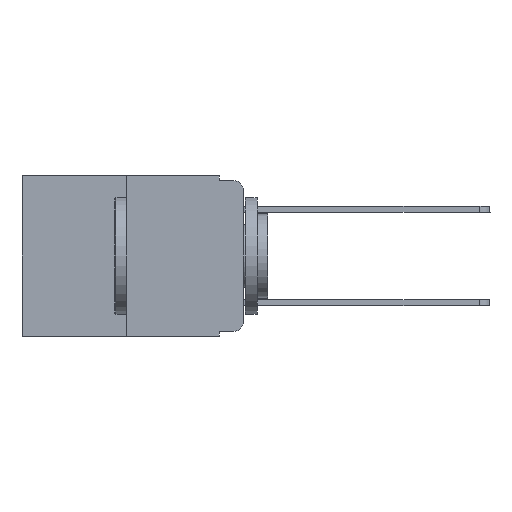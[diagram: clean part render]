
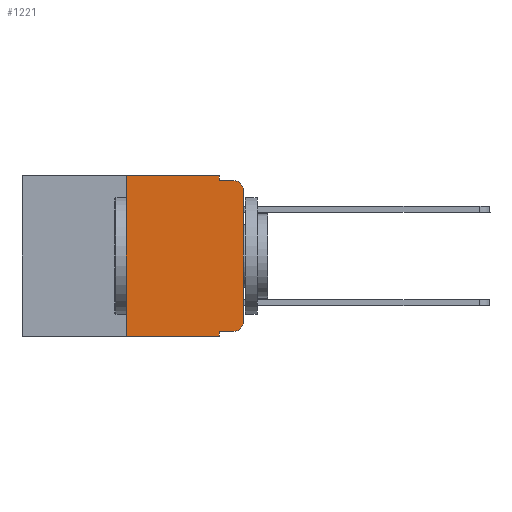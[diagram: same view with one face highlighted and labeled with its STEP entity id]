
A CAD part, left-side view. The second image highlights one B-rep face of the part: STEP entity #1221.
In plain terms, the highlighted planar face has unit normal (-1, 0, 0).
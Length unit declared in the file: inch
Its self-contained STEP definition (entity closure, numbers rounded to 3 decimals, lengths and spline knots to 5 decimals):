
#422 = AXIS2_PLACEMENT_3D ( 'NONE', #8731, #4426, #17679 ) ;
#542 = CARTESIAN_POINT ( 'NONE',  ( 0., 0.02, -0.333 ) ) ;
#1221 = ADVANCED_FACE ( 'NONE', ( #9738 ), #8747, .F. ) ;
#1279 = VERTEX_POINT ( 'NONE', #10726 ) ;
#1606 = CARTESIAN_POINT ( 'NONE',  ( 0., 0.473, -0.343 ) ) ;
#2159 = VERTEX_POINT ( 'NONE', #2429 ) ;
#2238 = ORIENTED_EDGE ( 'NONE', *, *, #3857, .T. ) ;
#2368 = DIRECTION ( 'NONE',  ( -1., 0., 0. ) ) ;
#2429 = CARTESIAN_POINT ( 'NONE',  ( 0., 0.051, -0.343 ) ) ;
#2742 = VERTEX_POINT ( 'NONE', #5523 ) ;
#2778 = LINE ( 'NONE', #15766, #17876 ) ;
#3284 = ORIENTED_EDGE ( 'NONE', *, *, #5958, .T. ) ;
#3495 = EDGE_CURVE ( 'NONE', #1279, #2742, #3902, .T. ) ;
#3747 = EDGE_CURVE ( 'NONE', #4686, #7341, #6860, .T. ) ;
#3857 = EDGE_CURVE ( 'NONE', #1279, #2159, #15197, .T. ) ;
#3902 = LINE ( 'NONE', #12713, #14790 ) ;
#4000 = ORIENTED_EDGE ( 'NONE', *, *, #8654, .F. ) ;
#4116 = VECTOR ( 'NONE', #4656, 39.37008 ) ;
#4294 = VECTOR ( 'NONE', #17960, 39.37008 ) ;
#4426 = DIRECTION ( 'NONE',  ( -1., 0., 0. ) ) ;
#4656 = DIRECTION ( 'NONE',  ( 0., 0., 1. ) ) ;
#4686 = VERTEX_POINT ( 'NONE', #17404 ) ;
#4939 = ORIENTED_EDGE ( 'NONE', *, *, #3747, .F. ) ;
#4977 = EDGE_LOOP ( 'NONE', ( #18023, #12356, #4939, #4000, #7674, #10097, #2238, #9635, #3284, #13152 ) ) ;
#5523 = CARTESIAN_POINT ( 'NONE',  ( 0., 0.25, 0. ) ) ;
#5594 = VECTOR ( 'NONE', #13557, 39.37008 ) ;
#5663 = DIRECTION ( 'NONE',  ( 0., -1., 0. ) ) ;
#5920 = VECTOR ( 'NONE', #16324, 39.37008 ) ;
#5958 = EDGE_CURVE ( 'NONE', #7833, #14600, #10935, .T. ) ;
#6187 = EDGE_CURVE ( 'NONE', #2742, #14765, #11849, .T. ) ;
#6364 = AXIS2_PLACEMENT_3D ( 'NONE', #13652, #2368, #8349 ) ;
#6860 = LINE ( 'NONE', #14422, #5920 ) ;
#7187 = CARTESIAN_POINT ( 'NONE',  ( 0., 0.473, 0. ) ) ;
#7341 = VERTEX_POINT ( 'NONE', #7884 ) ;
#7361 = DIRECTION ( 'NONE',  ( 1., 0., 0. ) ) ;
#7467 = EDGE_CURVE ( 'NONE', #7833, #2159, #2778, .T. ) ;
#7553 = CARTESIAN_POINT ( 'NONE',  ( 0., 0.051, -0.333 ) ) ;
#7674 = ORIENTED_EDGE ( 'NONE', *, *, #6187, .F. ) ;
#7833 = VERTEX_POINT ( 'NONE', #7553 ) ;
#7859 = CARTESIAN_POINT ( 'NONE',  ( 0., 0., -0.03 ) ) ;
#7884 = CARTESIAN_POINT ( 'NONE',  ( 0., 0.02, -0.01 ) ) ;
#8015 = LINE ( 'NONE', #14967, #4116 ) ;
#8028 = AXIS2_PLACEMENT_3D ( 'NONE', #7187, #7361, #16200 ) ;
#8089 = DIRECTION ( 'NONE',  ( 0., 0., 1. ) ) ;
#8349 = DIRECTION ( 'NONE',  ( 0., 0., -1. ) ) ;
#8575 = VECTOR ( 'NONE', #5663, 39.37008 ) ;
#8654 = EDGE_CURVE ( 'NONE', #14765, #4686, #13655, .T. ) ;
#8731 = CARTESIAN_POINT ( 'NONE',  ( 0., 0.02, -0.313 ) ) ;
#8747 = PLANE ( 'NONE',  #8028 ) ;
#9041 = CARTESIAN_POINT ( 'NONE',  ( 0., 0.473, 0. ) ) ;
#9262 = EDGE_CURVE ( 'NONE', #11565, #16363, #8015, .T. ) ;
#9635 = ORIENTED_EDGE ( 'NONE', *, *, #7467, .F. ) ;
#9666 = VECTOR ( 'NONE', #17744, 39.37008 ) ;
#9738 = FACE_OUTER_BOUND ( 'NONE', #4977, .T. ) ;
#10097 = ORIENTED_EDGE ( 'NONE', *, *, #3495, .F. ) ;
#10449 = CARTESIAN_POINT ( 'NONE',  ( 0., 0.051, 0. ) ) ;
#10726 = CARTESIAN_POINT ( 'NONE',  ( 0., 0.25, -0.343 ) ) ;
#10935 = LINE ( 'NONE', #19224, #8575 ) ;
#11143 = DIRECTION ( 'NONE',  ( 0., 0., -1. ) ) ;
#11505 = CARTESIAN_POINT ( 'NONE',  ( 0., 0.051, 0. ) ) ;
#11565 = VERTEX_POINT ( 'NONE', #15838 ) ;
#11849 = LINE ( 'NONE', #9041, #5594 ) ;
#12356 = ORIENTED_EDGE ( 'NONE', *, *, #12972, .T. ) ;
#12713 = CARTESIAN_POINT ( 'NONE',  ( 0., 0.25, 0. ) ) ;
#12972 = EDGE_CURVE ( 'NONE', #16363, #7341, #18394, .T. ) ;
#13152 = ORIENTED_EDGE ( 'NONE', *, *, #14836, .T. ) ;
#13557 = DIRECTION ( 'NONE',  ( 0., -1., 0. ) ) ;
#13652 = CARTESIAN_POINT ( 'NONE',  ( 0., 0.02, -0.03 ) ) ;
#13655 = LINE ( 'NONE', #10449, #9666 ) ;
#14422 = CARTESIAN_POINT ( 'NONE',  ( 0., 0.051, -0.01 ) ) ;
#14600 = VERTEX_POINT ( 'NONE', #542 ) ;
#14765 = VERTEX_POINT ( 'NONE', #11505 ) ;
#14790 = VECTOR ( 'NONE', #8089, 39.37008 ) ;
#14836 = EDGE_CURVE ( 'NONE', #14600, #11565, #15282, .T. ) ;
#14967 = CARTESIAN_POINT ( 'NONE',  ( 0., 0., 0. ) ) ;
#15197 = LINE ( 'NONE', #1606, #4294 ) ;
#15282 = CIRCLE ( 'NONE', #422, 0.02 ) ;
#15766 = CARTESIAN_POINT ( 'NONE',  ( 0., 0.051, 0. ) ) ;
#15838 = CARTESIAN_POINT ( 'NONE',  ( 0., 0., -0.313 ) ) ;
#16200 = DIRECTION ( 'NONE',  ( 0., 0., -1. ) ) ;
#16324 = DIRECTION ( 'NONE',  ( 0., -1., 0. ) ) ;
#16363 = VERTEX_POINT ( 'NONE', #7859 ) ;
#17404 = CARTESIAN_POINT ( 'NONE',  ( 0., 0.051, -0.01 ) ) ;
#17679 = DIRECTION ( 'NONE',  ( 0., 0., -1. ) ) ;
#17744 = DIRECTION ( 'NONE',  ( 0., 0., -1. ) ) ;
#17876 = VECTOR ( 'NONE', #11143, 39.37008 ) ;
#17960 = DIRECTION ( 'NONE',  ( 0., -1., 0. ) ) ;
#18023 = ORIENTED_EDGE ( 'NONE', *, *, #9262, .T. ) ;
#18394 = CIRCLE ( 'NONE', #6364, 0.02 ) ;
#19224 = CARTESIAN_POINT ( 'NONE',  ( 0., 0.051, -0.333 ) ) ;
